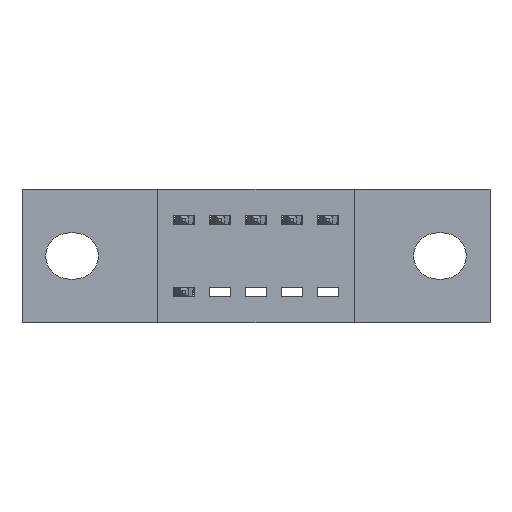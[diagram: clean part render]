
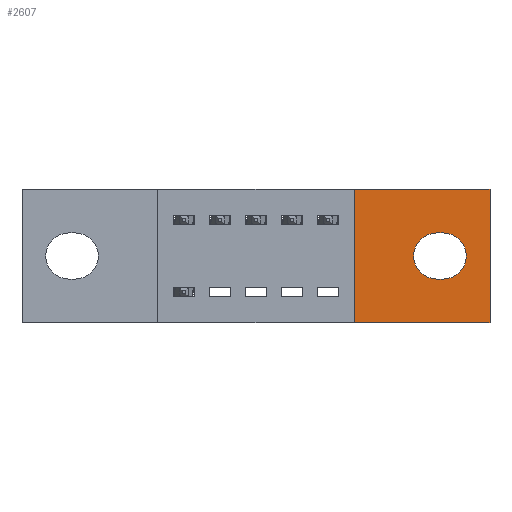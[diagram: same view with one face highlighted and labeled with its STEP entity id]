
A CAD part, front view. The second image highlights one B-rep face of the part: STEP entity #2607.
In plain terms, the highlighted planar face has unit normal (0, -1, 0).
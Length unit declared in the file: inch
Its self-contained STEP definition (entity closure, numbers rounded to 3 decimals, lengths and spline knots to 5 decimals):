
#127 = ORIENTED_EDGE ( 'NONE', *, *, #2711, .T. ) ;
#153 = DIRECTION ( 'NONE',  ( 0., 0., -1. ) ) ;
#160 = CARTESIAN_POINT ( 'NONE',  ( 1.3, 0., 0. ) ) ;
#301 = DIRECTION ( 'NONE',  ( 0., 1., 0. ) ) ;
#381 = DIRECTION ( 'NONE',  ( 1., 0., 0. ) ) ;
#387 = CARTESIAN_POINT ( 'NONE',  ( 1.17, 0., -0.185 ) ) ;
#448 = CARTESIAN_POINT ( 'NONE',  ( 1.152, 0., -0.185 ) ) ;
#581 = EDGE_CURVE ( 'NONE', #1504, #2030, #2388, .T. ) ;
#898 = LINE ( 'NONE', #2839, #5675 ) ;
#1011 = EDGE_CURVE ( 'NONE', #3584, #2085, #898, .T. ) ;
#1303 = VERTEX_POINT ( 'NONE', #4565 ) ;
#1315 = CIRCLE ( 'NONE', #6480, 0.064 ) ;
#1451 = VERTEX_POINT ( 'NONE', #5380 ) ;
#1470 = VERTEX_POINT ( 'NONE', #2339 ) ;
#1475 = CARTESIAN_POINT ( 'NONE',  ( 1.17, 0., -0.121 ) ) ;
#1504 = VERTEX_POINT ( 'NONE', #4677 ) ;
#1942 = EDGE_CURVE ( 'NONE', #2030, #5151, #5163, .T. ) ;
#2028 = LINE ( 'NONE', #3829, #2200 ) ;
#2030 = VERTEX_POINT ( 'NONE', #2900 ) ;
#2085 = VERTEX_POINT ( 'NONE', #1475 ) ;
#2133 = FACE_OUTER_BOUND ( 'NONE', #2162, .T. ) ;
#2162 = EDGE_LOOP ( 'NONE', ( #5340, #6884, #5714, #6089 ) ) ;
#2200 = VECTOR ( 'NONE', #2502, 39.37008 ) ;
#2339 = CARTESIAN_POINT ( 'NONE',  ( 1.17, 0., -0.249 ) ) ;
#2388 = LINE ( 'NONE', #5291, #6852 ) ;
#2502 = DIRECTION ( 'NONE',  ( -1., 0., 0. ) ) ;
#2607 = ADVANCED_FACE ( 'NONE', ( #5433, #2133 ), #5286, .T. ) ;
#2679 = DIRECTION ( 'NONE',  ( 1., 0., 0. ) ) ;
#2711 = EDGE_CURVE ( 'NONE', #1303, #3584, #1315, .T. ) ;
#2809 = CARTESIAN_POINT ( 'NONE',  ( 1.152, 0., -0.121 ) ) ;
#2839 = CARTESIAN_POINT ( 'NONE',  ( 1.17, 0., -0.121 ) ) ;
#2900 = CARTESIAN_POINT ( 'NONE',  ( 0.923, 0., 0. ) ) ;
#3066 = DIRECTION ( 'NONE',  ( 0., 0., -1. ) ) ;
#3137 = CARTESIAN_POINT ( 'NONE',  ( 0., 0., 0. ) ) ;
#3146 = VECTOR ( 'NONE', #381, 39.37008 ) ;
#3243 = AXIS2_PLACEMENT_3D ( 'NONE', #7213, #7178, #3066 ) ;
#3301 = VECTOR ( 'NONE', #5796, 39.37008 ) ;
#3306 = DIRECTION ( 'NONE',  ( 0., 1., 0. ) ) ;
#3441 = DIRECTION ( 'NONE',  ( -1., 0., 0. ) ) ;
#3456 = CARTESIAN_POINT ( 'NONE',  ( 0., 0., -0.37 ) ) ;
#3562 = EDGE_CURVE ( 'NONE', #1470, #1303, #2028, .T. ) ;
#3584 = VERTEX_POINT ( 'NONE', #2809 ) ;
#3829 = CARTESIAN_POINT ( 'NONE',  ( 1.17, 0., -0.249 ) ) ;
#3949 = EDGE_CURVE ( 'NONE', #2085, #1470, #5969, .T. ) ;
#4068 = CARTESIAN_POINT ( 'NONE',  ( 1.3, 0., 0. ) ) ;
#4282 = AXIS2_PLACEMENT_3D ( 'NONE', #387, #301, #153 ) ;
#4565 = CARTESIAN_POINT ( 'NONE',  ( 1.152, 0., -0.249 ) ) ;
#4677 = CARTESIAN_POINT ( 'NONE',  ( 0.923, 0., -0.37 ) ) ;
#4692 = LINE ( 'NONE', #3456, #4887 ) ;
#4887 = VECTOR ( 'NONE', #3441, 39.37008 ) ;
#5151 = VERTEX_POINT ( 'NONE', #4068 ) ;
#5152 = ORIENTED_EDGE ( 'NONE', *, *, #1011, .T. ) ;
#5163 = LINE ( 'NONE', #3137, #3146 ) ;
#5286 = PLANE ( 'NONE',  #3243 ) ;
#5291 = CARTESIAN_POINT ( 'NONE',  ( 0.923, 0., -0.37 ) ) ;
#5340 = ORIENTED_EDGE ( 'NONE', *, *, #581, .F. ) ;
#5380 = CARTESIAN_POINT ( 'NONE',  ( 1.3, 0., -0.37 ) ) ;
#5433 = FACE_BOUND ( 'NONE', #7070, .T. ) ;
#5675 = VECTOR ( 'NONE', #2679, 39.37008 ) ;
#5714 = ORIENTED_EDGE ( 'NONE', *, *, #7603, .F. ) ;
#5796 = DIRECTION ( 'NONE',  ( 0., 0., -1. ) ) ;
#5969 = CIRCLE ( 'NONE', #4282, 0.064 ) ;
#6089 = ORIENTED_EDGE ( 'NONE', *, *, #1942, .F. ) ;
#6170 = ORIENTED_EDGE ( 'NONE', *, *, #3949, .T. ) ;
#6345 = ORIENTED_EDGE ( 'NONE', *, *, #3562, .T. ) ;
#6480 = AXIS2_PLACEMENT_3D ( 'NONE', #448, #3306, #7785 ) ;
#6816 = EDGE_CURVE ( 'NONE', #1451, #1504, #4692, .T. ) ;
#6852 = VECTOR ( 'NONE', #7844, 39.37008 ) ;
#6860 = LINE ( 'NONE', #160, #3301 ) ;
#6884 = ORIENTED_EDGE ( 'NONE', *, *, #6816, .F. ) ;
#7070 = EDGE_LOOP ( 'NONE', ( #6170, #6345, #127, #5152 ) ) ;
#7178 = DIRECTION ( 'NONE',  ( 0., -1., 0. ) ) ;
#7213 = CARTESIAN_POINT ( 'NONE',  ( 0., 0., -0.37 ) ) ;
#7603 = EDGE_CURVE ( 'NONE', #5151, #1451, #6860, .T. ) ;
#7785 = DIRECTION ( 'NONE',  ( 0., 0., -1. ) ) ;
#7844 = DIRECTION ( 'NONE',  ( 0., 0., 1. ) ) ;
